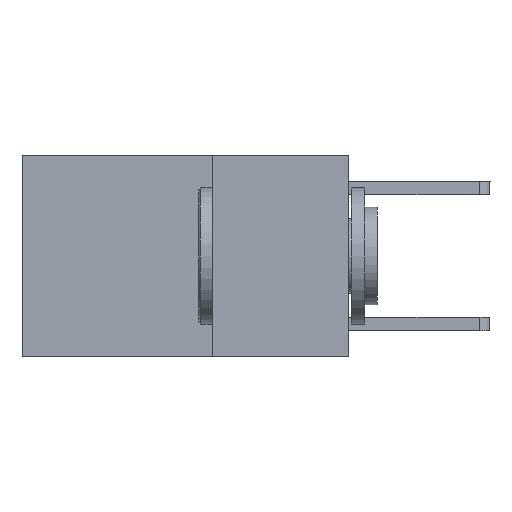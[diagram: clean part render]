
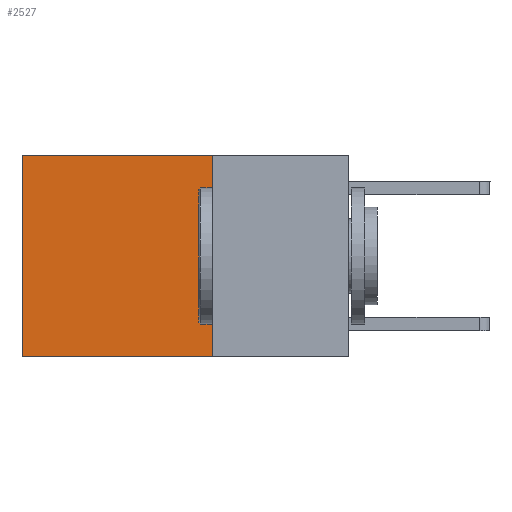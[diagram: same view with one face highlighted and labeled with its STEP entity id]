
A CAD part, left-side view. The second image highlights one B-rep face of the part: STEP entity #2527.
In plain terms, the highlighted planar face has unit normal (-1, 0, 0).
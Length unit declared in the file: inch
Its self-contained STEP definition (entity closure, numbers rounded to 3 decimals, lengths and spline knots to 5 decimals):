
#817 = DIRECTION ( 'NONE',  ( 0., 1., 0. ) ) ;
#1116 = VECTOR ( 'NONE', #817, 39.37008 ) ;
#1524 = VECTOR ( 'NONE', #4303, 39.37008 ) ;
#1719 = LINE ( 'NONE', #9210, #1524 ) ;
#1795 = VERTEX_POINT ( 'NONE', #8825 ) ;
#1922 = VECTOR ( 'NONE', #5820, 39.37008 ) ;
#2455 = LINE ( 'NONE', #7441, #1922 ) ;
#2527 = ADVANCED_FACE ( 'NONE', ( #3525 ), #3258, .F. ) ;
#2661 = EDGE_CURVE ( 'NONE', #9141, #5600, #1719, .T. ) ;
#3122 = CARTESIAN_POINT ( 'NONE',  ( 0.2625, 0.25, 0. ) ) ;
#3258 = PLANE ( 'NONE',  #4943 ) ;
#3267 = VERTEX_POINT ( 'NONE', #5038 ) ;
#3395 = DIRECTION ( 'NONE',  ( 1., 0., 0. ) ) ;
#3479 = DIRECTION ( 'NONE',  ( 0., 0., -1. ) ) ;
#3525 = FACE_OUTER_BOUND ( 'NONE', #8056, .T. ) ;
#3634 = ORIENTED_EDGE ( 'NONE', *, *, #5665, .T. ) ;
#3770 = ORIENTED_EDGE ( 'NONE', *, *, #6053, .F. ) ;
#3779 = LINE ( 'NONE', #4975, #7349 ) ;
#4303 = DIRECTION ( 'NONE',  ( 0., 0., -1. ) ) ;
#4920 = ORIENTED_EDGE ( 'NONE', *, *, #7403, .F. ) ;
#4943 = AXIS2_PLACEMENT_3D ( 'NONE', #3122, #3395, #3479 ) ;
#4975 = CARTESIAN_POINT ( 'NONE',  ( 0.2625, 0.25, 0. ) ) ;
#5038 = CARTESIAN_POINT ( 'NONE',  ( 0.2625, 0.25, 0. ) ) ;
#5600 = VERTEX_POINT ( 'NONE', #6525 ) ;
#5665 = EDGE_CURVE ( 'NONE', #3267, #9141, #2455, .T. ) ;
#5802 = ORIENTED_EDGE ( 'NONE', *, *, #2661, .T. ) ;
#5820 = DIRECTION ( 'NONE',  ( 0., 1., 0. ) ) ;
#6053 = EDGE_CURVE ( 'NONE', #1795, #5600, #9122, .T. ) ;
#6525 = CARTESIAN_POINT ( 'NONE',  ( 0.2625, 0.6, -0.37 ) ) ;
#7165 = CARTESIAN_POINT ( 'NONE',  ( 0.2625, 0.25, -0.37 ) ) ;
#7270 = DIRECTION ( 'NONE',  ( 0., 0., -1. ) ) ;
#7349 = VECTOR ( 'NONE', #7270, 39.37008 ) ;
#7403 = EDGE_CURVE ( 'NONE', #3267, #1795, #3779, .T. ) ;
#7441 = CARTESIAN_POINT ( 'NONE',  ( 0.2625, 0.25, 0. ) ) ;
#8056 = EDGE_LOOP ( 'NONE', ( #5802, #3770, #4920, #3634 ) ) ;
#8772 = CARTESIAN_POINT ( 'NONE',  ( 0.2625, 0.6, 0. ) ) ;
#8825 = CARTESIAN_POINT ( 'NONE',  ( 0.2625, 0.25, -0.37 ) ) ;
#9122 = LINE ( 'NONE', #7165, #1116 ) ;
#9141 = VERTEX_POINT ( 'NONE', #8772 ) ;
#9210 = CARTESIAN_POINT ( 'NONE',  ( 0.2625, 0.6, 0. ) ) ;
